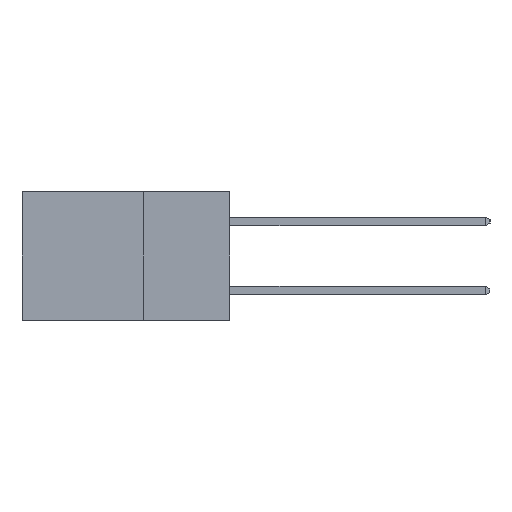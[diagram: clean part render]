
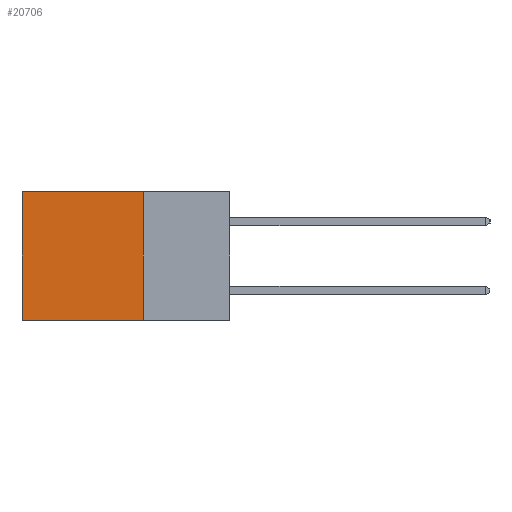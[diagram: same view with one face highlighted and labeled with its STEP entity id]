
A CAD part, left-side view. The second image highlights one B-rep face of the part: STEP entity #20706.
In plain terms, the highlighted planar face has unit normal (-1, 0, 0).
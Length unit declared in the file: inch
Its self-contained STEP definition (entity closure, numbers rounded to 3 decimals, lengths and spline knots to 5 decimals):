
#90 = CARTESIAN_POINT ( 'NONE',  ( 0.298, 0.6, 0. ) ) ;
#292 = VECTOR ( 'NONE', #6597, 39.37008 ) ;
#391 = ORIENTED_EDGE ( 'NONE', *, *, #22760, .T. ) ;
#1327 = LINE ( 'NONE', #7105, #15289 ) ;
#1657 = VECTOR ( 'NONE', #7645, 39.37008 ) ;
#2166 = EDGE_LOOP ( 'NONE', ( #391, #17202, #13966, #21171 ) ) ;
#2917 = DIRECTION ( 'NONE',  ( 0., 0., -1. ) ) ;
#3825 = LINE ( 'NONE', #22672, #21878 ) ;
#4865 = DIRECTION ( 'NONE',  ( 1., 0., 0. ) ) ;
#5134 = LINE ( 'NONE', #17519, #292 ) ;
#5806 = CARTESIAN_POINT ( 'NONE',  ( 0.298, 0.25, -0.37 ) ) ;
#6597 = DIRECTION ( 'NONE',  ( 0., 1., 0. ) ) ;
#7105 = CARTESIAN_POINT ( 'NONE',  ( 0.298, 0.6, 0. ) ) ;
#7645 = DIRECTION ( 'NONE',  ( 0., 1., 0. ) ) ;
#9508 = VERTEX_POINT ( 'NONE', #20695 ) ;
#10690 = FACE_OUTER_BOUND ( 'NONE', #2166, .T. ) ;
#11375 = VERTEX_POINT ( 'NONE', #90 ) ;
#11380 = LINE ( 'NONE', #5806, #1657 ) ;
#13358 = EDGE_CURVE ( 'NONE', #9508, #13823, #11380, .T. ) ;
#13823 = VERTEX_POINT ( 'NONE', #19581 ) ;
#13966 = ORIENTED_EDGE ( 'NONE', *, *, #15293, .F. ) ;
#15289 = VECTOR ( 'NONE', #21514, 39.37008 ) ;
#15293 = EDGE_CURVE ( 'NONE', #16741, #9508, #3825, .T. ) ;
#15792 = PLANE ( 'NONE',  #21995 ) ;
#16007 = EDGE_CURVE ( 'NONE', #16741, #11375, #5134, .T. ) ;
#16741 = VERTEX_POINT ( 'NONE', #21077 ) ;
#17202 = ORIENTED_EDGE ( 'NONE', *, *, #13358, .F. ) ;
#17519 = CARTESIAN_POINT ( 'NONE',  ( 0.298, 0.25, 0. ) ) ;
#17537 = CARTESIAN_POINT ( 'NONE',  ( 0.298, 0.25, 0. ) ) ;
#17613 = DIRECTION ( 'NONE',  ( 0., 0., -1. ) ) ;
#19581 = CARTESIAN_POINT ( 'NONE',  ( 0.298, 0.6, -0.37 ) ) ;
#20695 = CARTESIAN_POINT ( 'NONE',  ( 0.298, 0.25, -0.37 ) ) ;
#20706 = ADVANCED_FACE ( 'NONE', ( #10690 ), #15792, .F. ) ;
#21077 = CARTESIAN_POINT ( 'NONE',  ( 0.298, 0.25, 0. ) ) ;
#21171 = ORIENTED_EDGE ( 'NONE', *, *, #16007, .T. ) ;
#21514 = DIRECTION ( 'NONE',  ( 0., 0., -1. ) ) ;
#21878 = VECTOR ( 'NONE', #2917, 39.37008 ) ;
#21995 = AXIS2_PLACEMENT_3D ( 'NONE', #17537, #4865, #17613 ) ;
#22672 = CARTESIAN_POINT ( 'NONE',  ( 0.298, 0.25, 0. ) ) ;
#22760 = EDGE_CURVE ( 'NONE', #11375, #13823, #1327, .T. ) ;
